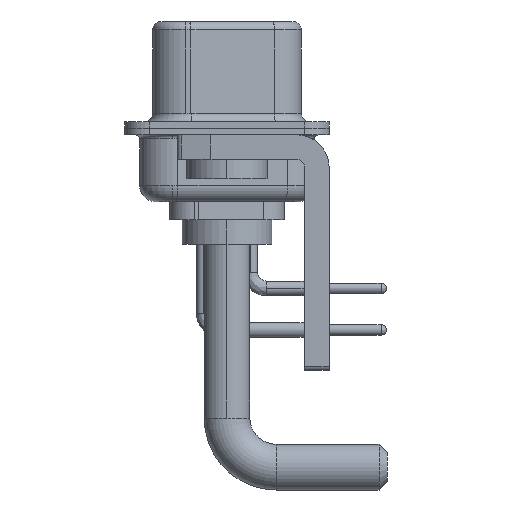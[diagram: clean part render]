
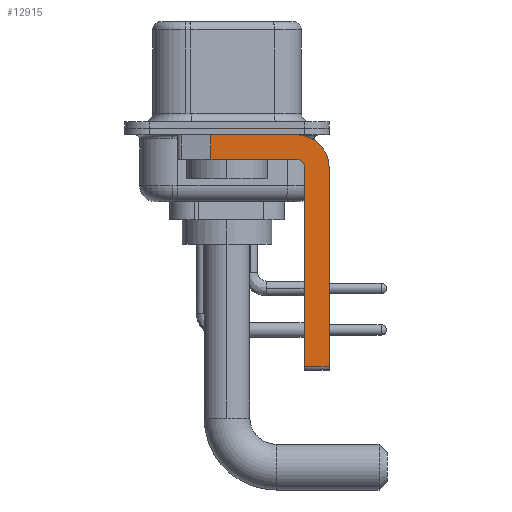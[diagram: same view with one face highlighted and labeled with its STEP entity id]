
A CAD part, left-side view. The second image highlights one B-rep face of the part: STEP entity #12915.
In plain terms, the highlighted planar face has unit normal (-1, 0, 0).
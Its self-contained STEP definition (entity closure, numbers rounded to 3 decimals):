
#411 = AXIS2_PLACEMENT_3D ( 'NONE', #15559, #9744, #7582 ) ;
#758 = DIRECTION ( 'NONE',  ( 1., 0., 0. ) ) ;
#1881 = CARTESIAN_POINT ( 'NONE',  ( -2.9, -6.25, -2.4 ) ) ;
#1941 = CARTESIAN_POINT ( 'NONE',  ( -2.9, 0.978, -0.4 ) ) ;
#2045 = VECTOR ( 'NONE', #10358, 1000. ) ;
#2321 = VERTEX_POINT ( 'NONE', #4903 ) ;
#2494 = EDGE_CURVE ( 'NONE', #4736, #19060, #19332, .T. ) ;
#2686 = CARTESIAN_POINT ( 'NONE',  ( -2.9, -6.25, -2.4 ) ) ;
#3073 = LINE ( 'NONE', #16862, #8559 ) ;
#3318 = CARTESIAN_POINT ( 'NONE',  ( -2.9, -4.25, -2.4 ) ) ;
#4736 = VERTEX_POINT ( 'NONE', #1941 ) ;
#4903 = CARTESIAN_POINT ( 'NONE',  ( -2.9, -4.25, -1.9 ) ) ;
#5005 = CIRCLE ( 'NONE', #17782, 0.5 ) ;
#5824 = VERTEX_POINT ( 'NONE', #2686 ) ;
#6008 = ORIENTED_EDGE ( 'NONE', *, *, #2494, .F. ) ;
#6508 = VERTEX_POINT ( 'NONE', #21294 ) ;
#6761 = CARTESIAN_POINT ( 'NONE',  ( -2.9, -4.75, -14.55 ) ) ;
#7091 = VERTEX_POINT ( 'NONE', #13569 ) ;
#7582 = DIRECTION ( 'NONE',  ( 0., 0., -1. ) ) ;
#7676 = LINE ( 'NONE', #1881, #12782 ) ;
#7875 = LINE ( 'NONE', #25362, #17934 ) ;
#8251 = EDGE_CURVE ( 'NONE', #24480, #6508, #3073, .T. ) ;
#8559 = VECTOR ( 'NONE', #19030, 1000. ) ;
#9304 = EDGE_CURVE ( 'NONE', #24480, #21727, #7875, .T. ) ;
#9366 = FACE_OUTER_BOUND ( 'NONE', #19279, .T. ) ;
#9539 = DIRECTION ( 'NONE',  ( 0., -1., 0. ) ) ;
#9744 = DIRECTION ( 'NONE',  ( 1., 0., 0. ) ) ;
#10226 = LINE ( 'NONE', #24002, #2045 ) ;
#10358 = DIRECTION ( 'NONE',  ( 0., 0., -1. ) ) ;
#11706 = ORIENTED_EDGE ( 'NONE', *, *, #9304, .F. ) ;
#11719 = DIRECTION ( 'NONE',  ( 0., 0., 1. ) ) ;
#12782 = VECTOR ( 'NONE', #15540, 1000. ) ;
#12915 = ADVANCED_FACE ( 'NONE', ( #9366 ), #15701, .F. ) ;
#13151 = CARTESIAN_POINT ( 'NONE',  ( -2.9, 3., -0.4 ) ) ;
#13219 = DIRECTION ( 'NONE',  ( -1., 0., 0. ) ) ;
#13569 = CARTESIAN_POINT ( 'NONE',  ( -2.9, 0.978, -1.9 ) ) ;
#13601 = EDGE_CURVE ( 'NONE', #4736, #7091, #10226, .T. ) ;
#13806 = DIRECTION ( 'NONE',  ( 0., 1., 0. ) ) ;
#13839 = ORIENTED_EDGE ( 'NONE', *, *, #15782, .F. ) ;
#13992 = VECTOR ( 'NONE', #13806, 1000. ) ;
#14393 = CARTESIAN_POINT ( 'NONE',  ( -2.9, -4.25, -2.4 ) ) ;
#15540 = DIRECTION ( 'NONE',  ( 0., 0., -1. ) ) ;
#15559 = CARTESIAN_POINT ( 'NONE',  ( -2.9, -4.25, -2.4 ) ) ;
#15649 = LINE ( 'NONE', #21165, #13992 ) ;
#15701 = PLANE ( 'NONE',  #411 ) ;
#15782 = EDGE_CURVE ( 'NONE', #19060, #5824, #16087, .T. ) ;
#16087 = CIRCLE ( 'NONE', #22662, 2. ) ;
#16125 = EDGE_CURVE ( 'NONE', #5824, #6508, #7676, .T. ) ;
#16862 = CARTESIAN_POINT ( 'NONE',  ( -2.9, -4.25, -14.55 ) ) ;
#17138 = EDGE_CURVE ( 'NONE', #21727, #2321, #5005, .T. ) ;
#17782 = AXIS2_PLACEMENT_3D ( 'NONE', #3318, #13219, #23255 ) ;
#17934 = VECTOR ( 'NONE', #11719, 1000. ) ;
#18164 = ORIENTED_EDGE ( 'NONE', *, *, #13601, .T. ) ;
#18751 = DIRECTION ( 'NONE',  ( 0., 0., -1. ) ) ;
#19030 = DIRECTION ( 'NONE',  ( 0., -1., 0. ) ) ;
#19060 = VERTEX_POINT ( 'NONE', #21686 ) ;
#19279 = EDGE_LOOP ( 'NONE', ( #6008, #18164, #21471, #22190, #11706, #20738, #20228, #13839 ) ) ;
#19295 = VECTOR ( 'NONE', #9539, 1000. ) ;
#19332 = LINE ( 'NONE', #13151, #19295 ) ;
#20228 = ORIENTED_EDGE ( 'NONE', *, *, #16125, .F. ) ;
#20738 = ORIENTED_EDGE ( 'NONE', *, *, #8251, .T. ) ;
#21165 = CARTESIAN_POINT ( 'NONE',  ( -2.9, -4.25, -1.9 ) ) ;
#21294 = CARTESIAN_POINT ( 'NONE',  ( -2.9, -6.25, -14.55 ) ) ;
#21471 = ORIENTED_EDGE ( 'NONE', *, *, #24738, .F. ) ;
#21686 = CARTESIAN_POINT ( 'NONE',  ( -2.9, -4.25, -0.4 ) ) ;
#21727 = VERTEX_POINT ( 'NONE', #22735 ) ;
#22190 = ORIENTED_EDGE ( 'NONE', *, *, #17138, .F. ) ;
#22662 = AXIS2_PLACEMENT_3D ( 'NONE', #14393, #758, #18751 ) ;
#22735 = CARTESIAN_POINT ( 'NONE',  ( -2.9, -4.75, -2.4 ) ) ;
#23255 = DIRECTION ( 'NONE',  ( 0., 0., 1. ) ) ;
#24002 = CARTESIAN_POINT ( 'NONE',  ( -2.9, 0.978, -1.9 ) ) ;
#24480 = VERTEX_POINT ( 'NONE', #6761 ) ;
#24738 = EDGE_CURVE ( 'NONE', #2321, #7091, #15649, .T. ) ;
#25362 = CARTESIAN_POINT ( 'NONE',  ( -2.9, -4.75, -14.8 ) ) ;
